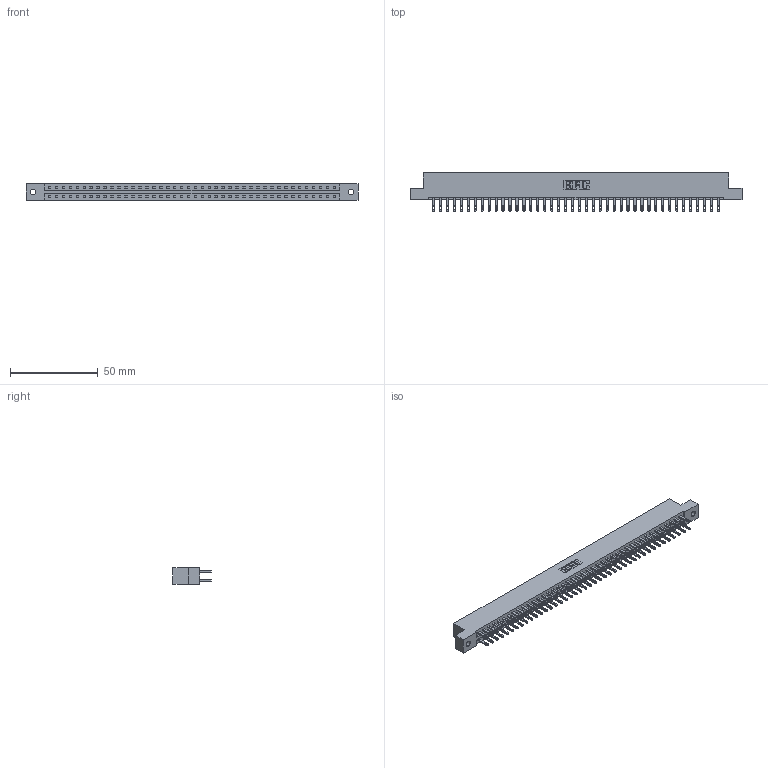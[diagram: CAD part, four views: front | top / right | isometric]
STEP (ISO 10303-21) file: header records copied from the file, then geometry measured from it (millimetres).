
FILE_DESCRIPTION (( 'STEP AP203' ), '1' );
FILE_NAME ('337-084-500-202.STEP', '2018-08-12T21:38:06', ( '' ), ( '' ), 'SwSTEP 2.0', 'SolidWorks 2016', '' );
FILE_SCHEMA (( 'CONFIG_CONTROL_DESIGN' ));
Length unit declared in the file: inch
Products named in the file (3): 337 Part_Flush Mounting Lugs - 0.128 Dia; 345-292-001_345-293-100; 337-084-500-202
Assembly tree (85 placements, depth 2):
  337-084-500-202
    337 Part_Flush Mounting Lugs - 0.128 Dia
    345-292-001_345-293-100  x84
Bounding box: 189.43 x 21.85 x 9.4 mm (x, y, z)
Volume: 20184 mm3; surface area: 23477.4 mm2
Topology: 85 solids, 85 shells, 4314 faces, 13163 edges, 8774 vertices
Faces by surface type: plane 2758, cylinder 1556
Entity records: 32497 total; most frequent: CARTESIAN_POINT 5474, ORIENTED_EDGE 5410, DIRECTION 4657, EDGE_CURVE 2705, VECTOR 2573, LINE 2573, VERTEX_POINT 1802, AXIS2_PLACEMENT_3D 1042
